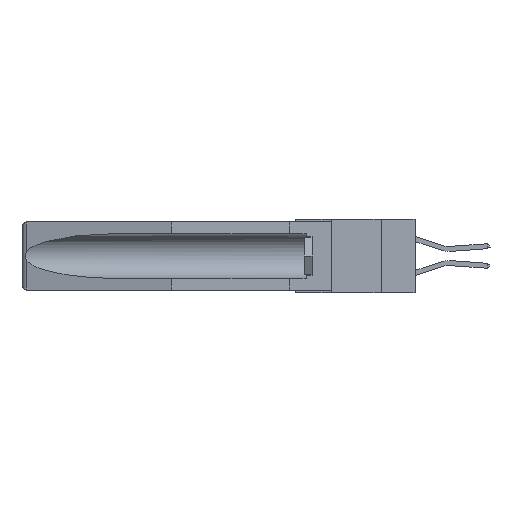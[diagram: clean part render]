
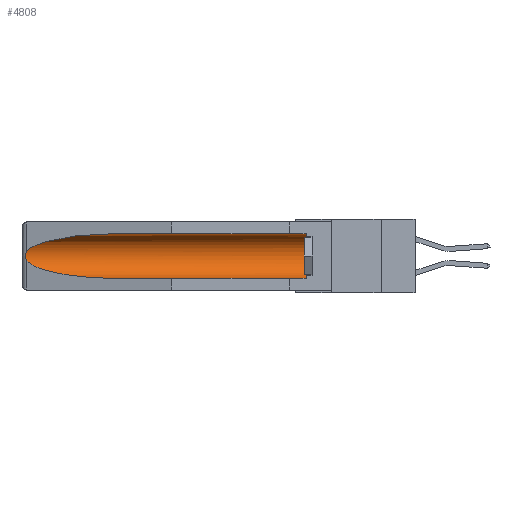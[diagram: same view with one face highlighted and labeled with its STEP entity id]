
A CAD part, left-side view. The second image highlights one B-rep face of the part: STEP entity #4808.
In plain terms, the highlighted cylindrical face has radius 2.857 mm (diameter 5.715 mm), a partial arc.
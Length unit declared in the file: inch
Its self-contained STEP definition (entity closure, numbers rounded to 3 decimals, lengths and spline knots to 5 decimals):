
#391 = CARTESIAN_POINT ( 'NONE',  ( 0.25451, 1.48313, -0.24835 ) ) ;
#1181 = CARTESIAN_POINT ( 'NONE',  ( 0.2673, 1.5327, -0.16383 ) ) ;
#1510 = LINE ( 'NONE', #8150, #3778 ) ;
#1634 = EDGE_CURVE ( 'NONE', #16391, #1780, #16472, .T. ) ;
#1780 = VERTEX_POINT ( 'NONE', #20157 ) ;
#1793 = CYLINDRICAL_SURFACE ( 'NONE', #8795, 0.1125 ) ;
#2272 = CARTESIAN_POINT ( 'NONE',  ( 0.26537, 1.52718, -0.19328 ) ) ;
#2345 = DIRECTION ( 'NONE',  ( 0., 1., 0. ) ) ;
#2779 = CARTESIAN_POINT ( 'NONE',  ( 0.25451, 1.48313, -0.09465 ) ) ;
#3122 = CARTESIAN_POINT ( 'NONE',  ( 0.26654, 1.53092, -0.15636 ) ) ;
#3182 = EDGE_CURVE ( 'NONE', #11305, #16391, #5670, .T. ) ;
#3778 = VECTOR ( 'NONE', #2345, 39.37008 ) ;
#3881 = VECTOR ( 'NONE', #12490, 39.37008 ) ;
#4767 = ORIENTED_EDGE ( 'NONE', *, *, #16786, .T. ) ;
#4808 = ADVANCED_FACE ( 'NONE', ( #7062 ), #1793, .F. ) ;
#5590 = CARTESIAN_POINT ( 'NONE',  ( 0.26537, 1.52718, -0.19328 ) ) ;
#5670 = LINE ( 'NONE', #8968, #3881 ) ;
#6626 = EDGE_CURVE ( 'NONE', #22926, #20160, #1510, .T. ) ;
#6881 = CARTESIAN_POINT ( 'NONE',  ( 0.2675, 1.53308, -0.16763 ) ) ;
#7062 = FACE_OUTER_BOUND ( 'NONE', #12077, .T. ) ;
#7791 =( BOUNDED_CURVE ( )  B_SPLINE_CURVE ( 3, ( #2272, #391, #11743, #11819 ),
 .UNSPECIFIED., .F., .F. ) 
 B_SPLINE_CURVE_WITH_KNOTS ( ( 4, 4 ),
 ( 0.1948, 1.5708 ),
 .UNSPECIFIED. ) 
 CURVE ( )  GEOMETRIC_REPRESENTATION_ITEM ( )  RATIONAL_B_SPLINE_CURVE ( ( 1., 0.848, 0.848, 1. ) ) 
 REPRESENTATION_ITEM ( '' )  );
#8118 = ORIENTED_EDGE ( 'NONE', *, *, #1634, .T. ) ;
#8150 = CARTESIAN_POINT ( 'NONE',  ( 0.155, -0.30754, -0.284 ) ) ;
#8396 = EDGE_CURVE ( 'NONE', #1780, #24140, #21602, .T. ) ;
#8695 = CARTESIAN_POINT ( 'NONE',  ( 0.26655, 1.53094, -0.18657 ) ) ;
#8795 = AXIS2_PLACEMENT_3D ( 'NONE', #18396, #23809, #12565 ) ;
#8968 = CARTESIAN_POINT ( 'NONE',  ( 0.155, -0.30754, -0.059 ) ) ;
#10789 = CARTESIAN_POINT ( 'NONE',  ( 0.155, 0.126, -0.059 ) ) ;
#11305 = VERTEX_POINT ( 'NONE', #10789 ) ;
#11399 = ORIENTED_EDGE ( 'NONE', *, *, #8396, .T. ) ;
#11738 = AXIS2_PLACEMENT_3D ( 'NONE', #14114, #21677, #17978 ) ;
#11743 = CARTESIAN_POINT ( 'NONE',  ( 0.21114, 1.30732, -0.284 ) ) ;
#11819 = CARTESIAN_POINT ( 'NONE',  ( 0.155, 1.07973, -0.284 ) ) ;
#12077 = EDGE_LOOP ( 'NONE', ( #8118, #11399, #20530, #16151, #4767, #19221 ) ) ;
#12179 = CARTESIAN_POINT ( 'NONE',  ( 0.21114, 1.30732, -0.059 ) ) ;
#12490 = DIRECTION ( 'NONE',  ( 0., 1., 0. ) ) ;
#12565 = DIRECTION ( 'NONE',  ( 0., 0., 1. ) ) ;
#12685 = CARTESIAN_POINT ( 'NONE',  ( 0.155, 0.126, -0.284 ) ) ;
#13722 = CARTESIAN_POINT ( 'NONE',  ( 0.26537, 1.52718, -0.14972 ) ) ;
#14114 = CARTESIAN_POINT ( 'NONE',  ( 0.155, 0.126, -0.1715 ) ) ;
#14145 = CARTESIAN_POINT ( 'NONE',  ( 0.26537, 1.52718, -0.19328 ) ) ;
#14956 = EDGE_CURVE ( 'NONE', #24140, #20160, #7791, .T. ) ;
#16151 = ORIENTED_EDGE ( 'NONE', *, *, #6626, .F. ) ;
#16207 = CARTESIAN_POINT ( 'NONE',  ( 0.2675, 1.53308, -0.17534 ) ) ;
#16391 = VERTEX_POINT ( 'NONE', #16601 ) ;
#16472 =( BOUNDED_CURVE ( )  B_SPLINE_CURVE ( 3, ( #21286, #12179, #2779, #13722 ),
 .UNSPECIFIED., .F., .F. ) 
 B_SPLINE_CURVE_WITH_KNOTS ( ( 4, 4 ),
 ( 4.71239, 6.08839 ),
 .UNSPECIFIED. ) 
 CURVE ( )  GEOMETRIC_REPRESENTATION_ITEM ( )  RATIONAL_B_SPLINE_CURVE ( ( 1., 0.848, 0.848, 1. ) ) 
 REPRESENTATION_ITEM ( '' )  );
#16601 = CARTESIAN_POINT ( 'NONE',  ( 0.155, 1.07973, -0.059 ) ) ;
#16786 = EDGE_CURVE ( 'NONE', #22926, #11305, #18637, .T. ) ;
#17978 = DIRECTION ( 'NONE',  ( 0., 0., 1. ) ) ;
#18012 = CARTESIAN_POINT ( 'NONE',  ( 0.26597, 1.5296, -0.19026 ) ) ;
#18102 = CARTESIAN_POINT ( 'NONE',  ( 0.2673, 1.53269, -0.17917 ) ) ;
#18396 = CARTESIAN_POINT ( 'NONE',  ( 0.155, -0.30754, -0.1715 ) ) ;
#18637 = CIRCLE ( 'NONE', #11738, 0.1125 ) ;
#19221 = ORIENTED_EDGE ( 'NONE', *, *, #3182, .T. ) ;
#19920 = CARTESIAN_POINT ( 'NONE',  ( 0.26537, 1.52718, -0.14972 ) ) ;
#20157 = CARTESIAN_POINT ( 'NONE',  ( 0.26537, 1.52718, -0.14972 ) ) ;
#20160 = VERTEX_POINT ( 'NONE', #23012 ) ;
#20530 = ORIENTED_EDGE ( 'NONE', *, *, #14956, .T. ) ;
#21286 = CARTESIAN_POINT ( 'NONE',  ( 0.155, 1.07973, -0.059 ) ) ;
#21602 = B_SPLINE_CURVE_WITH_KNOTS ( 'NONE', 3,
 ( #19920, #21964, #3122, #1181, #6881, #16207, #18102, #8695, #18012, #14145 ),
 .UNSPECIFIED., .F., .F.,
 ( 4, 2, 2, 2, 4 ),
 ( 0., 0.00029, 0.00058, 0.00087, 0.00117 ),
 .UNSPECIFIED. ) ;
#21677 = DIRECTION ( 'NONE',  ( 0., -1., 0. ) ) ;
#21964 = CARTESIAN_POINT ( 'NONE',  ( 0.26597, 1.52961, -0.15275 ) ) ;
#22926 = VERTEX_POINT ( 'NONE', #12685 ) ;
#23012 = CARTESIAN_POINT ( 'NONE',  ( 0.155, 1.07973, -0.284 ) ) ;
#23809 = DIRECTION ( 'NONE',  ( 0., 1., 0. ) ) ;
#24140 = VERTEX_POINT ( 'NONE', #5590 ) ;
